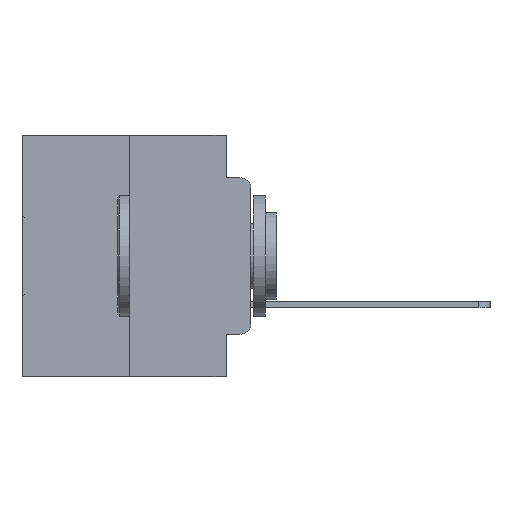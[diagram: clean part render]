
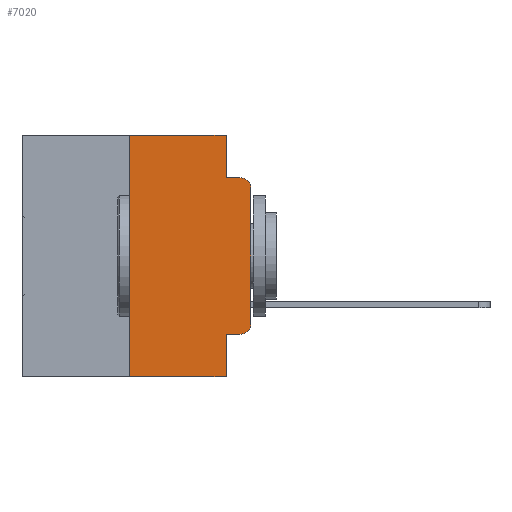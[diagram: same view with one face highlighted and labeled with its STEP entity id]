
A CAD part, left-side view. The second image highlights one B-rep face of the part: STEP entity #7020.
In plain terms, the highlighted planar face has unit normal (-1, 0, 0).
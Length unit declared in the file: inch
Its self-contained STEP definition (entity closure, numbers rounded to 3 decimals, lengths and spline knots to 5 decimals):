
#1893 = VECTOR ( 'NONE', #7984, 39.37008 ) ;
#1926 = EDGE_CURVE ( 'NONE', #8279, #31720, #5037, .T. ) ;
#2355 = AXIS2_PLACEMENT_3D ( 'NONE', #19375, #7247, #9365 ) ;
#2916 = DIRECTION ( 'NONE',  ( 0., 0., 1. ) ) ;
#3121 = CARTESIAN_POINT ( 'NONE',  ( 0., 0., -0.3915 ) ) ;
#3205 = EDGE_CURVE ( 'NONE', #8078, #16465, #6525, .T. ) ;
#3370 = VECTOR ( 'NONE', #7479, 39.37008 ) ;
#3411 = CIRCLE ( 'NONE', #31769, 0.02 ) ;
#3927 = CARTESIAN_POINT ( 'NONE',  ( 0., 0.02, -0.0885 ) ) ;
#4489 = ORIENTED_EDGE ( 'NONE', *, *, #10120, .T. ) ;
#5037 = LINE ( 'NONE', #24432, #3370 ) ;
#5321 = CARTESIAN_POINT ( 'NONE',  ( 0., 0.25, 0. ) ) ;
#6131 = VECTOR ( 'NONE', #6606, 39.37008 ) ;
#6525 = CIRCLE ( 'NONE', #17884, 0.02 ) ;
#6606 = DIRECTION ( 'NONE',  ( 0., -1., 0. ) ) ;
#6982 = CARTESIAN_POINT ( 'NONE',  ( 0., 0.051, 0. ) ) ;
#7020 = ADVANCED_FACE ( 'NONE', ( #26799 ), #14508, .F. ) ;
#7247 = DIRECTION ( 'NONE',  ( 1., 0., 0. ) ) ;
#7278 = ORIENTED_EDGE ( 'NONE', *, *, #22408, .F. ) ;
#7315 = DIRECTION ( 'NONE',  ( -1., 0., 0. ) ) ;
#7479 = DIRECTION ( 'NONE',  ( 0., -1., 0. ) ) ;
#7728 = ORIENTED_EDGE ( 'NONE', *, *, #13512, .F. ) ;
#7984 = DIRECTION ( 'NONE',  ( 0., 0., 1. ) ) ;
#8078 = VERTEX_POINT ( 'NONE', #15658 ) ;
#8279 = VERTEX_POINT ( 'NONE', #17103 ) ;
#8698 = CARTESIAN_POINT ( 'NONE',  ( 0., 0.051, -0.4115 ) ) ;
#9365 = DIRECTION ( 'NONE',  ( 0., 0., -1. ) ) ;
#9497 = CARTESIAN_POINT ( 'NONE',  ( 0., 0.02, -0.3915 ) ) ;
#9716 = EDGE_CURVE ( 'NONE', #27964, #15069, #12584, .T. ) ;
#10120 = EDGE_CURVE ( 'NONE', #30216, #21030, #3411, .T. ) ;
#10695 = EDGE_CURVE ( 'NONE', #21030, #8078, #30098, .T. ) ;
#11134 = CARTESIAN_POINT ( 'NONE',  ( 0., 0.051, -0.4115 ) ) ;
#11424 = ORIENTED_EDGE ( 'NONE', *, *, #18401, .F. ) ;
#11582 = CARTESIAN_POINT ( 'NONE',  ( 0., 0.051, 0. ) ) ;
#12164 = DIRECTION ( 'NONE',  ( 0., 0., -1. ) ) ;
#12584 = LINE ( 'NONE', #20498, #15407 ) ;
#12641 = DIRECTION ( 'NONE',  ( 0., 0., -1. ) ) ;
#12824 = CARTESIAN_POINT ( 'NONE',  ( 0., 0., 0. ) ) ;
#12991 = CARTESIAN_POINT ( 'NONE',  ( 0., 0.051, -0.5 ) ) ;
#13179 = ORIENTED_EDGE ( 'NONE', *, *, #9716, .T. ) ;
#13512 = EDGE_CURVE ( 'NONE', #31720, #25061, #26547, .T. ) ;
#14362 = EDGE_CURVE ( 'NONE', #27009, #15069, #17709, .T. ) ;
#14363 = VECTOR ( 'NONE', #17071, 39.37008 ) ;
#14492 = VECTOR ( 'NONE', #2916, 39.37008 ) ;
#14508 = PLANE ( 'NONE',  #2355 ) ;
#15069 = VERTEX_POINT ( 'NONE', #12991 ) ;
#15407 = VECTOR ( 'NONE', #24697, 39.37008 ) ;
#15658 = CARTESIAN_POINT ( 'NONE',  ( 0., 0., -0.1085 ) ) ;
#16465 = VERTEX_POINT ( 'NONE', #3927 ) ;
#17071 = DIRECTION ( 'NONE',  ( 0., 0., -1. ) ) ;
#17103 = CARTESIAN_POINT ( 'NONE',  ( 0., 0.25, 0. ) ) ;
#17704 = DIRECTION ( 'NONE',  ( 0., 0., -1. ) ) ;
#17709 = LINE ( 'NONE', #29670, #14363 ) ;
#17884 = AXIS2_PLACEMENT_3D ( 'NONE', #22044, #7315, #12641 ) ;
#18068 = ORIENTED_EDGE ( 'NONE', *, *, #10695, .T. ) ;
#18401 = EDGE_CURVE ( 'NONE', #27964, #8279, #27465, .T. ) ;
#18899 = LINE ( 'NONE', #28738, #6131 ) ;
#19194 = CARTESIAN_POINT ( 'NONE',  ( 0., 0.051, -0.0885 ) ) ;
#19345 = DIRECTION ( 'NONE',  ( -1., 0., 0. ) ) ;
#19375 = CARTESIAN_POINT ( 'NONE',  ( 0., 0.473, 0. ) ) ;
#20159 = ORIENTED_EDGE ( 'NONE', *, *, #29754, .T. ) ;
#20498 = CARTESIAN_POINT ( 'NONE',  ( 0., 0.473, -0.5 ) ) ;
#20987 = LINE ( 'NONE', #8698, #29586 ) ;
#21030 = VERTEX_POINT ( 'NONE', #3121 ) ;
#22044 = CARTESIAN_POINT ( 'NONE',  ( 0., 0.02, -0.1085 ) ) ;
#22408 = EDGE_CURVE ( 'NONE', #25061, #16465, #18899, .T. ) ;
#23560 = DIRECTION ( 'NONE',  ( 0., -1., 0. ) ) ;
#23681 = ORIENTED_EDGE ( 'NONE', *, *, #3205, .T. ) ;
#24139 = VECTOR ( 'NONE', #12164, 39.37008 ) ;
#24432 = CARTESIAN_POINT ( 'NONE',  ( 0., 0.473, 0. ) ) ;
#24697 = DIRECTION ( 'NONE',  ( 0., -1., 0. ) ) ;
#25061 = VERTEX_POINT ( 'NONE', #19194 ) ;
#25355 = ORIENTED_EDGE ( 'NONE', *, *, #1926, .F. ) ;
#26547 = LINE ( 'NONE', #6982, #24139 ) ;
#26799 = FACE_OUTER_BOUND ( 'NONE', #31394, .T. ) ;
#27009 = VERTEX_POINT ( 'NONE', #11134 ) ;
#27465 = LINE ( 'NONE', #5321, #14492 ) ;
#27964 = VERTEX_POINT ( 'NONE', #28964 ) ;
#28738 = CARTESIAN_POINT ( 'NONE',  ( 0., 0.051, -0.0885 ) ) ;
#28964 = CARTESIAN_POINT ( 'NONE',  ( 0., 0.25, -0.5 ) ) ;
#29205 = CARTESIAN_POINT ( 'NONE',  ( 0., 0.02, -0.4115 ) ) ;
#29586 = VECTOR ( 'NONE', #23560, 39.37008 ) ;
#29667 = ORIENTED_EDGE ( 'NONE', *, *, #14362, .F. ) ;
#29670 = CARTESIAN_POINT ( 'NONE',  ( 0., 0.051, 0. ) ) ;
#29754 = EDGE_CURVE ( 'NONE', #27009, #30216, #20987, .T. ) ;
#30098 = LINE ( 'NONE', #12824, #1893 ) ;
#30216 = VERTEX_POINT ( 'NONE', #29205 ) ;
#31394 = EDGE_LOOP ( 'NONE', ( #18068, #23681, #7278, #7728, #25355, #11424, #13179, #29667, #20159, #4489 ) ) ;
#31720 = VERTEX_POINT ( 'NONE', #11582 ) ;
#31769 = AXIS2_PLACEMENT_3D ( 'NONE', #9497, #19345, #17704 ) ;
